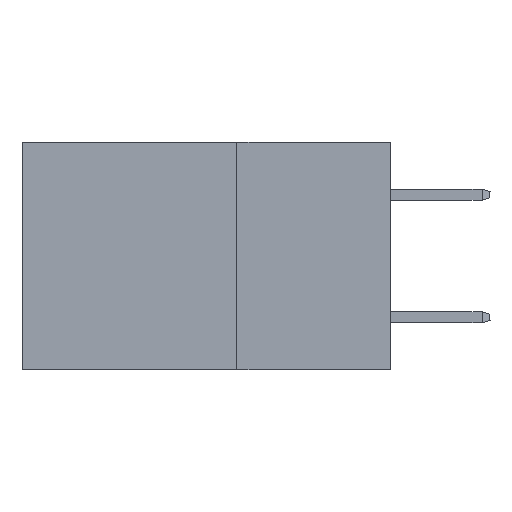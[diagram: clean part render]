
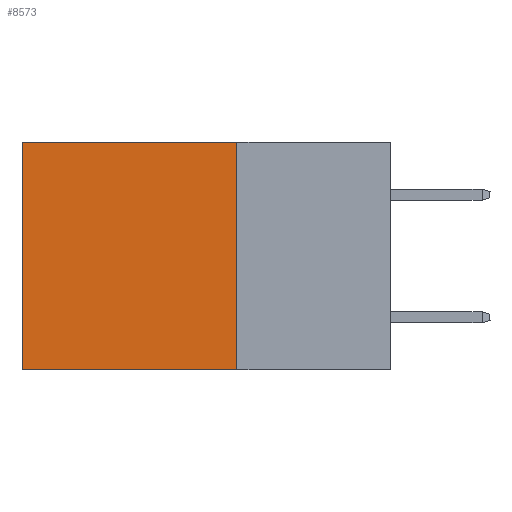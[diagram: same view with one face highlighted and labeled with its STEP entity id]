
A CAD part, left-side view. The second image highlights one B-rep face of the part: STEP entity #8573.
In plain terms, the highlighted planar face has unit normal (-1, 0, 0).
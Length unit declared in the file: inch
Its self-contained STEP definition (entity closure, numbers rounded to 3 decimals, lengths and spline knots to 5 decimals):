
#850 = DIRECTION ( 'NONE',  ( 0., 1., 0. ) ) ;
#899 = LINE ( 'NONE', #24715, #31394 ) ;
#1088 = VERTEX_POINT ( 'NONE', #18639 ) ;
#1335 = EDGE_LOOP ( 'NONE', ( #35383, #37236, #16869, #22061 ) ) ;
#2438 = EDGE_CURVE ( 'NONE', #32015, #10107, #899, .T. ) ;
#5288 = LINE ( 'NONE', #30398, #31589 ) ;
#5871 = DIRECTION ( 'NONE',  ( 1., 0., 0. ) ) ;
#8573 = ADVANCED_FACE ( 'NONE', ( #14142 ), #25687, .F. ) ;
#9072 = EDGE_CURVE ( 'NONE', #32015, #28836, #28292, .T. ) ;
#10107 = VERTEX_POINT ( 'NONE', #33599 ) ;
#10823 = DIRECTION ( 'NONE',  ( 0., 0., -1. ) ) ;
#13691 = LINE ( 'NONE', #23931, #30802 ) ;
#14142 = FACE_OUTER_BOUND ( 'NONE', #1335, .T. ) ;
#14284 = AXIS2_PLACEMENT_3D ( 'NONE', #17306, #5871, #32154 ) ;
#14602 = CARTESIAN_POINT ( 'NONE',  ( 0.2875, 0.25, -0.37 ) ) ;
#15628 = EDGE_CURVE ( 'NONE', #28836, #1088, #13691, .T. ) ;
#15787 = DIRECTION ( 'NONE',  ( 0., 0., -1. ) ) ;
#16869 = ORIENTED_EDGE ( 'NONE', *, *, #9072, .F. ) ;
#17306 = CARTESIAN_POINT ( 'NONE',  ( 0.2875, 0.25, 0. ) ) ;
#17904 = EDGE_CURVE ( 'NONE', #10107, #1088, #5288, .T. ) ;
#18578 = VECTOR ( 'NONE', #10823, 39.37008 ) ;
#18639 = CARTESIAN_POINT ( 'NONE',  ( 0.2875, 0.6, -0.37 ) ) ;
#22061 = ORIENTED_EDGE ( 'NONE', *, *, #2438, .T. ) ;
#23931 = CARTESIAN_POINT ( 'NONE',  ( 0.2875, 0.25, -0.37 ) ) ;
#24715 = CARTESIAN_POINT ( 'NONE',  ( 0.2875, 0.25, 0. ) ) ;
#24773 = CARTESIAN_POINT ( 'NONE',  ( 0.2875, 0.25, 0. ) ) ;
#25687 = PLANE ( 'NONE',  #14284 ) ;
#28292 = LINE ( 'NONE', #37530, #18578 ) ;
#28836 = VERTEX_POINT ( 'NONE', #14602 ) ;
#30398 = CARTESIAN_POINT ( 'NONE',  ( 0.2875, 0.6, 0. ) ) ;
#30802 = VECTOR ( 'NONE', #850, 39.37008 ) ;
#31394 = VECTOR ( 'NONE', #36278, 39.37008 ) ;
#31589 = VECTOR ( 'NONE', #15787, 39.37008 ) ;
#32015 = VERTEX_POINT ( 'NONE', #24773 ) ;
#32154 = DIRECTION ( 'NONE',  ( 0., 0., -1. ) ) ;
#33599 = CARTESIAN_POINT ( 'NONE',  ( 0.2875, 0.6, 0. ) ) ;
#35383 = ORIENTED_EDGE ( 'NONE', *, *, #17904, .T. ) ;
#36278 = DIRECTION ( 'NONE',  ( 0., 1., 0. ) ) ;
#37236 = ORIENTED_EDGE ( 'NONE', *, *, #15628, .F. ) ;
#37530 = CARTESIAN_POINT ( 'NONE',  ( 0.2875, 0.25, 0. ) ) ;
